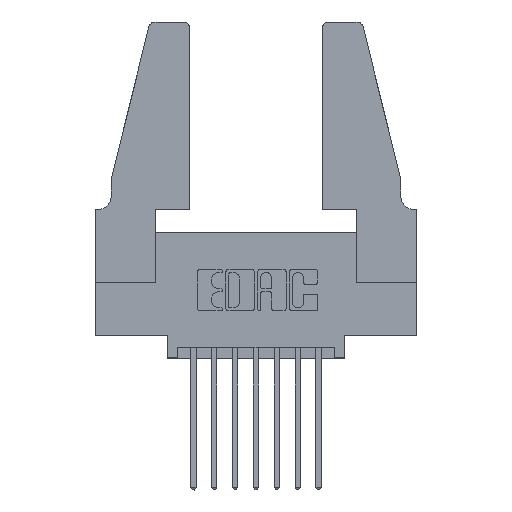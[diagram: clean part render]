
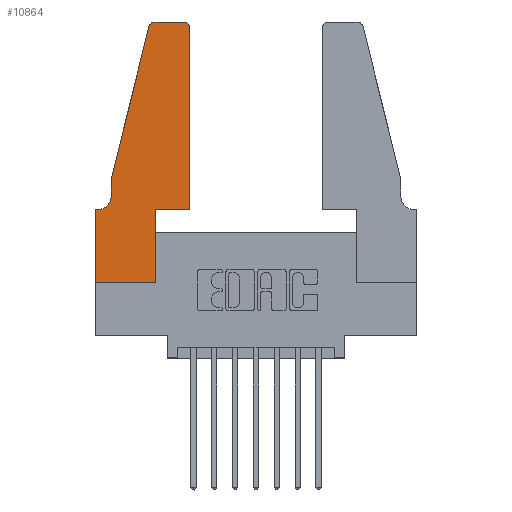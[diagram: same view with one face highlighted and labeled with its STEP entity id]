
A CAD part, top view. The second image highlights one B-rep face of the part: STEP entity #10864.
In plain terms, the highlighted planar face has unit normal (0, 0, 1).
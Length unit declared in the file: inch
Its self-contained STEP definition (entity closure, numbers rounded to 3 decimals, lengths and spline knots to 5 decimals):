
#212 = CARTESIAN_POINT ( 'NONE',  ( 0., 0., 0.37 ) ) ;
#254 = DIRECTION ( 'NONE',  ( 1., 0., 0. ) ) ;
#298 = LINE ( 'NONE', #9771, #5896 ) ;
#409 = CARTESIAN_POINT ( 'NONE',  ( 0.4505, 0.35, 0.37 ) ) ;
#559 = CARTESIAN_POINT ( 'NONE',  ( 0.2865, 0., 0.37 ) ) ;
#1009 = VERTEX_POINT ( 'NONE', #9383 ) ;
#1094 = EDGE_CURVE ( 'NONE', #2436, #1009, #5134, .T. ) ;
#1379 = DIRECTION ( 'NONE',  ( 1., 0., 0. ) ) ;
#1453 = VECTOR ( 'NONE', #2039, 39.37008 ) ;
#1514 = ORIENTED_EDGE ( 'NONE', *, *, #5830, .T. ) ;
#1686 = EDGE_CURVE ( 'NONE', #3063, #9342, #12085, .T. ) ;
#1945 = EDGE_CURVE ( 'NONE', #10539, #12228, #298, .T. ) ;
#2039 = DIRECTION ( 'NONE',  ( 0., 1., 0. ) ) ;
#2087 = EDGE_CURVE ( 'NONE', #2711, #2970, #6185, .T. ) ;
#2139 = ORIENTED_EDGE ( 'NONE', *, *, #7505, .T. ) ;
#2145 = ORIENTED_EDGE ( 'NONE', *, *, #1945, .T. ) ;
#2436 = VERTEX_POINT ( 'NONE', #9672 ) ;
#2512 = VECTOR ( 'NONE', #10450, 39.37008 ) ;
#2643 = DIRECTION ( 'NONE',  ( 0., 0., 1. ) ) ;
#2711 = VERTEX_POINT ( 'NONE', #3818 ) ;
#2970 = VERTEX_POINT ( 'NONE', #3156 ) ;
#2984 = VERTEX_POINT ( 'NONE', #559 ) ;
#3063 = VERTEX_POINT ( 'NONE', #12452 ) ;
#3130 = LINE ( 'NONE', #212, #8745 ) ;
#3156 = CARTESIAN_POINT ( 'NONE',  ( 0.284, 1.25, 0.37 ) ) ;
#3288 = DIRECTION ( 'NONE',  ( 0., 0., 1. ) ) ;
#3456 = EDGE_CURVE ( 'NONE', #1009, #4321, #8576, .T. ) ;
#3651 = EDGE_CURVE ( 'NONE', #2970, #2436, #6307, .T. ) ;
#3795 = EDGE_CURVE ( 'NONE', #9342, #7938, #10836, .T. ) ;
#3818 = CARTESIAN_POINT ( 'NONE',  ( 0.4205, 1.25, 0.37 ) ) ;
#4039 = DIRECTION ( 'NONE',  ( 0., 0., -1. ) ) ;
#4321 = VERTEX_POINT ( 'NONE', #12444 ) ;
#4426 = VECTOR ( 'NONE', #9570, 39.37008 ) ;
#4603 = CARTESIAN_POINT ( 'NONE',  ( 0.4505, 0.35, 0.37 ) ) ;
#4669 = PLANE ( 'NONE',  #12507 ) ;
#4768 = ORIENTED_EDGE ( 'NONE', *, *, #2087, .T. ) ;
#5134 = LINE ( 'NONE', #9781, #10604 ) ;
#5615 = EDGE_CURVE ( 'NONE', #7938, #2711, #10657, .T. ) ;
#5716 = CARTESIAN_POINT ( 'NONE',  ( 0.2865, 0.35, 0.37 ) ) ;
#5816 = DIRECTION ( 'NONE',  ( 1., 0., 0. ) ) ;
#5821 = DIRECTION ( 'NONE',  ( -1., 0., 0. ) ) ;
#5830 = EDGE_CURVE ( 'NONE', #4321, #10539, #11248, .T. ) ;
#5893 = ORIENTED_EDGE ( 'NONE', *, *, #3795, .T. ) ;
#5896 = VECTOR ( 'NONE', #5821, 39.37008 ) ;
#6065 = VECTOR ( 'NONE', #8728, 39.37008 ) ;
#6185 = LINE ( 'NONE', #6515, #11783 ) ;
#6195 = DIRECTION ( 'NONE',  ( 1., 0., 0. ) ) ;
#6237 = CARTESIAN_POINT ( 'NONE',  ( 0.0055, 0.35, 0.37 ) ) ;
#6258 = CARTESIAN_POINT ( 'NONE',  ( 0.284, 1.22, 0.37 ) ) ;
#6307 = CIRCLE ( 'NONE', #11798, 0.03 ) ;
#6515 = CARTESIAN_POINT ( 'NONE',  ( 0.2605, 1.25, 0.37 ) ) ;
#6567 = DIRECTION ( 'NONE',  ( 1., 0., 0. ) ) ;
#7043 = EDGE_LOOP ( 'NONE', ( #4768, #11777, #11020, #8312, #1514, #2145, #10372, #2139, #11575, #9235, #5893, #11332 ) ) ;
#7099 = LINE ( 'NONE', #5716, #6065 ) ;
#7290 = AXIS2_PLACEMENT_3D ( 'NONE', #11232, #2643, #6567 ) ;
#7505 = EDGE_CURVE ( 'NONE', #12048, #2984, #3130, .T. ) ;
#7938 = VERTEX_POINT ( 'NONE', #11929 ) ;
#7944 = CARTESIAN_POINT ( 'NONE',  ( 0.0055, 0.42, 0.37 ) ) ;
#8312 = ORIENTED_EDGE ( 'NONE', *, *, #3456, .T. ) ;
#8576 = LINE ( 'NONE', #10360, #2512 ) ;
#8728 = DIRECTION ( 'NONE',  ( 0., 1., 0. ) ) ;
#8737 = CARTESIAN_POINT ( 'NONE',  ( 0., 0., 0.37 ) ) ;
#8745 = VECTOR ( 'NONE', #254, 39.37008 ) ;
#8935 = DIRECTION ( 'NONE',  ( -1., 0., 0. ) ) ;
#9063 = VECTOR ( 'NONE', #6195, 39.37008 ) ;
#9235 = ORIENTED_EDGE ( 'NONE', *, *, #1686, .T. ) ;
#9284 = CARTESIAN_POINT ( 'NONE',  ( 0., 0., 0.37 ) ) ;
#9342 = VERTEX_POINT ( 'NONE', #4603 ) ;
#9383 = CARTESIAN_POINT ( 'NONE',  ( 0.0755, 0.5, 0.37 ) ) ;
#9570 = DIRECTION ( 'NONE',  ( 0., -1., 0. ) ) ;
#9672 = CARTESIAN_POINT ( 'NONE',  ( 0.25487, 1.22718, 0.37 ) ) ;
#9771 = CARTESIAN_POINT ( 'NONE',  ( 0.0755, 0.35, 0.37 ) ) ;
#9781 = CARTESIAN_POINT ( 'NONE',  ( 0.0755, 0.5, 0.37 ) ) ;
#10360 = CARTESIAN_POINT ( 'NONE',  ( 0.0755, 0.5, 0.37 ) ) ;
#10372 = ORIENTED_EDGE ( 'NONE', *, *, #10775, .T. ) ;
#10412 = DIRECTION ( 'NONE',  ( -1., 0., 0. ) ) ;
#10450 = DIRECTION ( 'NONE',  ( 0., -1., 0. ) ) ;
#10539 = VERTEX_POINT ( 'NONE', #6237 ) ;
#10579 = CARTESIAN_POINT ( 'NONE',  ( 0.4505, 0.35, 0.37 ) ) ;
#10604 = VECTOR ( 'NONE', #10773, 39.37008 ) ;
#10657 = CIRCLE ( 'NONE', #7290, 0.03 ) ;
#10773 = DIRECTION ( 'NONE',  ( -0.239, -0.971, 0. ) ) ;
#10775 = EDGE_CURVE ( 'NONE', #12228, #12048, #12286, .T. ) ;
#10836 = LINE ( 'NONE', #10579, #1453 ) ;
#10864 = ADVANCED_FACE ( 'NONE', ( #11836 ), #4669, .T. ) ;
#11020 = ORIENTED_EDGE ( 'NONE', *, *, #1094, .T. ) ;
#11232 = CARTESIAN_POINT ( 'NONE',  ( 0.4205, 1.22, 0.37 ) ) ;
#11248 = CIRCLE ( 'NONE', #11662, 0.07 ) ;
#11332 = ORIENTED_EDGE ( 'NONE', *, *, #5615, .T. ) ;
#11548 = CARTESIAN_POINT ( 'NONE',  ( 0., 0.35, 0.37 ) ) ;
#11575 = ORIENTED_EDGE ( 'NONE', *, *, #12319, .T. ) ;
#11602 = DIRECTION ( 'NONE',  ( 0., 0., 1. ) ) ;
#11662 = AXIS2_PLACEMENT_3D ( 'NONE', #7944, #4039, #8935 ) ;
#11777 = ORIENTED_EDGE ( 'NONE', *, *, #3651, .T. ) ;
#11783 = VECTOR ( 'NONE', #10412, 39.37008 ) ;
#11798 = AXIS2_PLACEMENT_3D ( 'NONE', #6258, #3288, #1379 ) ;
#11836 = FACE_OUTER_BOUND ( 'NONE', #7043, .T. ) ;
#11929 = CARTESIAN_POINT ( 'NONE',  ( 0.4505, 1.22, 0.37 ) ) ;
#12048 = VERTEX_POINT ( 'NONE', #9284 ) ;
#12085 = LINE ( 'NONE', #409, #9063 ) ;
#12228 = VERTEX_POINT ( 'NONE', #12403 ) ;
#12286 = LINE ( 'NONE', #8737, #4426 ) ;
#12319 = EDGE_CURVE ( 'NONE', #2984, #3063, #7099, .T. ) ;
#12403 = CARTESIAN_POINT ( 'NONE',  ( 0., 0.35, 0.37 ) ) ;
#12444 = CARTESIAN_POINT ( 'NONE',  ( 0.0755, 0.42, 0.37 ) ) ;
#12452 = CARTESIAN_POINT ( 'NONE',  ( 0.2865, 0.35, 0.37 ) ) ;
#12507 = AXIS2_PLACEMENT_3D ( 'NONE', #11548, #11602, #5816 ) ;
